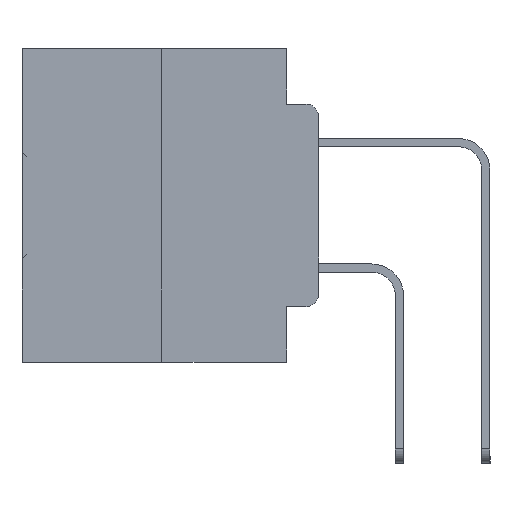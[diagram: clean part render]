
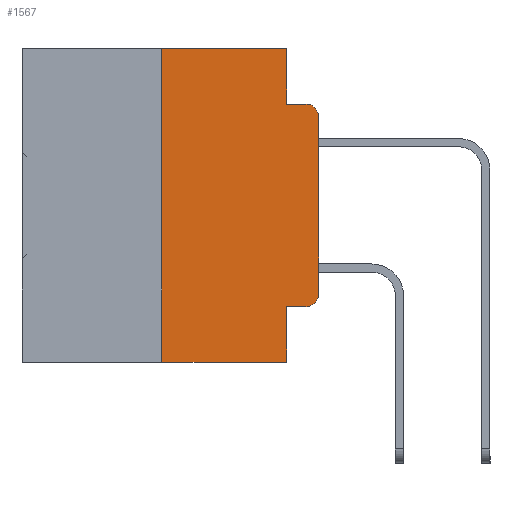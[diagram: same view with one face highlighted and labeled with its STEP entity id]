
A CAD part, left-side view. The second image highlights one B-rep face of the part: STEP entity #1567.
In plain terms, the highlighted planar face has unit normal (-1, 0, 0).
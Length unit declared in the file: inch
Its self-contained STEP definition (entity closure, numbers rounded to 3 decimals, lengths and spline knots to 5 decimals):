
#98 = VECTOR ( 'NONE', #13822, 39.37008 ) ;
#481 = DIRECTION ( 'NONE',  ( 0., -1., 0. ) ) ;
#1389 = DIRECTION ( 'NONE',  ( 0., 0., -1. ) ) ;
#1510 = LINE ( 'NONE', #22031, #15746 ) ;
#1567 = ADVANCED_FACE ( 'NONE', ( #20973 ), #14987, .F. ) ;
#2756 = VERTEX_POINT ( 'NONE', #14654 ) ;
#2980 = CARTESIAN_POINT ( 'NONE',  ( 0., 0., -0.1085 ) ) ;
#3031 = LINE ( 'NONE', #20440, #32174 ) ;
#3510 = CARTESIAN_POINT ( 'NONE',  ( 0., 0.02, -0.3915 ) ) ;
#5080 = VERTEX_POINT ( 'NONE', #12319 ) ;
#6517 = EDGE_CURVE ( 'NONE', #33185, #12872, #30797, .T. ) ;
#6557 = VERTEX_POINT ( 'NONE', #15401 ) ;
#6935 = DIRECTION ( 'NONE',  ( 0., 0., -1. ) ) ;
#7148 = ORIENTED_EDGE ( 'NONE', *, *, #18102, .T. ) ;
#7624 = CARTESIAN_POINT ( 'NONE',  ( 0., 0.473, 0. ) ) ;
#7842 = EDGE_CURVE ( 'NONE', #22484, #14494, #14748, .T. ) ;
#8918 = ORIENTED_EDGE ( 'NONE', *, *, #11063, .F. ) ;
#9382 = CARTESIAN_POINT ( 'NONE',  ( 0., 0.473, 0. ) ) ;
#9685 = CARTESIAN_POINT ( 'NONE',  ( 0., 0., -0.3915 ) ) ;
#10002 = EDGE_CURVE ( 'NONE', #10222, #12564, #36423, .T. ) ;
#10222 = VERTEX_POINT ( 'NONE', #13144 ) ;
#10542 = CARTESIAN_POINT ( 'NONE',  ( 0., 0.25, 0. ) ) ;
#10717 = VECTOR ( 'NONE', #19411, 39.37008 ) ;
#11063 = EDGE_CURVE ( 'NONE', #30115, #14494, #31239, .T. ) ;
#12319 = CARTESIAN_POINT ( 'NONE',  ( 0., 0.25, -0.5 ) ) ;
#12564 = VERTEX_POINT ( 'NONE', #14060 ) ;
#12872 = VERTEX_POINT ( 'NONE', #9685 ) ;
#13144 = CARTESIAN_POINT ( 'NONE',  ( 0., 0.051, -0.4115 ) ) ;
#13229 = ORIENTED_EDGE ( 'NONE', *, *, #16708, .T. ) ;
#13306 = DIRECTION ( 'NONE',  ( 0., 0., 1. ) ) ;
#13822 = DIRECTION ( 'NONE',  ( 0., -1., 0. ) ) ;
#14060 = CARTESIAN_POINT ( 'NONE',  ( 0., 0.051, -0.5 ) ) ;
#14072 = VECTOR ( 'NONE', #31793, 39.37008 ) ;
#14494 = VERTEX_POINT ( 'NONE', #30769 ) ;
#14654 = CARTESIAN_POINT ( 'NONE',  ( 0., 0.25, 0. ) ) ;
#14748 = CIRCLE ( 'NONE', #18462, 0.02 ) ;
#14923 = ORIENTED_EDGE ( 'NONE', *, *, #18933, .F. ) ;
#14987 = PLANE ( 'NONE',  #30118 ) ;
#15401 = CARTESIAN_POINT ( 'NONE',  ( 0., 0.051, 0. ) ) ;
#15746 = VECTOR ( 'NONE', #24768, 39.37008 ) ;
#16263 = VECTOR ( 'NONE', #28777, 39.37008 ) ;
#16423 = CARTESIAN_POINT ( 'NONE',  ( 0., 0.051, -0.0885 ) ) ;
#16708 = EDGE_CURVE ( 'NONE', #12872, #22484, #25818, .T. ) ;
#16899 = LINE ( 'NONE', #10542, #24483 ) ;
#16905 = ORIENTED_EDGE ( 'NONE', *, *, #25057, .F. ) ;
#17094 = LINE ( 'NONE', #25211, #98 ) ;
#17490 = AXIS2_PLACEMENT_3D ( 'NONE', #3510, #23405, #6935 ) ;
#17884 = DIRECTION ( 'NONE',  ( 0., 0., -1. ) ) ;
#17954 = EDGE_LOOP ( 'NONE', ( #13229, #25746, #8918, #36034, #14923, #16905, #7148, #25020, #33954, #21607 ) ) ;
#18102 = EDGE_CURVE ( 'NONE', #5080, #12564, #3031, .T. ) ;
#18427 = DIRECTION ( 'NONE',  ( -1., 0., 0. ) ) ;
#18462 = AXIS2_PLACEMENT_3D ( 'NONE', #35139, #18427, #1389 ) ;
#18933 = EDGE_CURVE ( 'NONE', #2756, #6557, #26523, .T. ) ;
#18955 = VECTOR ( 'NONE', #32906, 39.37008 ) ;
#19411 = DIRECTION ( 'NONE',  ( 0., 0., 1. ) ) ;
#20440 = CARTESIAN_POINT ( 'NONE',  ( 0., 0.473, -0.5 ) ) ;
#20973 = FACE_OUTER_BOUND ( 'NONE', #17954, .T. ) ;
#21607 = ORIENTED_EDGE ( 'NONE', *, *, #6517, .T. ) ;
#22031 = CARTESIAN_POINT ( 'NONE',  ( 0., 0.051, 0. ) ) ;
#22484 = VERTEX_POINT ( 'NONE', #2980 ) ;
#23405 = DIRECTION ( 'NONE',  ( -1., 0., 0. ) ) ;
#23972 = CARTESIAN_POINT ( 'NONE',  ( 0., 0.02, -0.4115 ) ) ;
#24483 = VECTOR ( 'NONE', #13306, 39.37008 ) ;
#24768 = DIRECTION ( 'NONE',  ( 0., 0., -1. ) ) ;
#24933 = EDGE_CURVE ( 'NONE', #10222, #33185, #17094, .T. ) ;
#25020 = ORIENTED_EDGE ( 'NONE', *, *, #10002, .F. ) ;
#25057 = EDGE_CURVE ( 'NONE', #5080, #2756, #16899, .T. ) ;
#25211 = CARTESIAN_POINT ( 'NONE',  ( 0., 0.051, -0.4115 ) ) ;
#25746 = ORIENTED_EDGE ( 'NONE', *, *, #7842, .T. ) ;
#25818 = LINE ( 'NONE', #33320, #10717 ) ;
#25955 = CARTESIAN_POINT ( 'NONE',  ( 0., 0.051, -0.0885 ) ) ;
#26382 = CARTESIAN_POINT ( 'NONE',  ( 0., 0.051, 0. ) ) ;
#26523 = LINE ( 'NONE', #7624, #18955 ) ;
#28777 = DIRECTION ( 'NONE',  ( 0., -1., 0. ) ) ;
#29792 = EDGE_CURVE ( 'NONE', #6557, #30115, #1510, .T. ) ;
#30115 = VERTEX_POINT ( 'NONE', #16423 ) ;
#30118 = AXIS2_PLACEMENT_3D ( 'NONE', #9382, #34612, #17884 ) ;
#30769 = CARTESIAN_POINT ( 'NONE',  ( 0., 0.02, -0.0885 ) ) ;
#30797 = CIRCLE ( 'NONE', #17490, 0.02 ) ;
#31239 = LINE ( 'NONE', #25955, #16263 ) ;
#31793 = DIRECTION ( 'NONE',  ( 0., 0., -1. ) ) ;
#32174 = VECTOR ( 'NONE', #481, 39.37008 ) ;
#32906 = DIRECTION ( 'NONE',  ( 0., -1., 0. ) ) ;
#33185 = VERTEX_POINT ( 'NONE', #23972 ) ;
#33320 = CARTESIAN_POINT ( 'NONE',  ( 0., 0., 0. ) ) ;
#33954 = ORIENTED_EDGE ( 'NONE', *, *, #24933, .T. ) ;
#34612 = DIRECTION ( 'NONE',  ( 1., 0., 0. ) ) ;
#35139 = CARTESIAN_POINT ( 'NONE',  ( 0., 0.02, -0.1085 ) ) ;
#36034 = ORIENTED_EDGE ( 'NONE', *, *, #29792, .F. ) ;
#36423 = LINE ( 'NONE', #26382, #14072 ) ;
